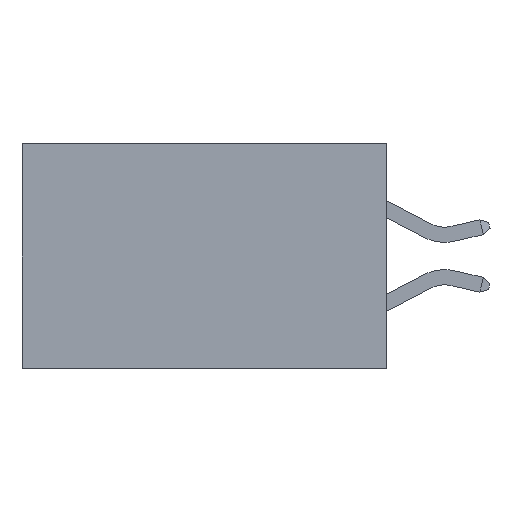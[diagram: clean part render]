
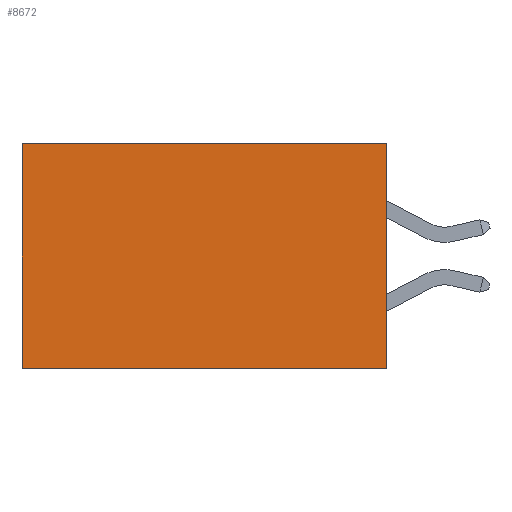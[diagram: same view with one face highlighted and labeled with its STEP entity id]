
A CAD part, left-side view. The second image highlights one B-rep face of the part: STEP entity #8672.
In plain terms, the highlighted planar face has unit normal (-1, 0, 0).
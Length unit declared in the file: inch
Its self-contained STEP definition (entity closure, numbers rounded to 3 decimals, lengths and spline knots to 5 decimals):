
#946 = EDGE_CURVE ( 'NONE', #15210, #5547, #4296, .T. ) ;
#956 = CARTESIAN_POINT ( 'NONE',  ( 0.2615, 0., -0.37 ) ) ;
#988 = DIRECTION ( 'NONE',  ( 0., 1., 0. ) ) ;
#1098 = VECTOR ( 'NONE', #13714, 39.37008 ) ;
#1459 = VERTEX_POINT ( 'NONE', #13126 ) ;
#1573 = CARTESIAN_POINT ( 'NONE',  ( 0.2615, 0., 0. ) ) ;
#2180 = LINE ( 'NONE', #15734, #11172 ) ;
#2649 = EDGE_CURVE ( 'NONE', #1459, #5547, #2180, .T. ) ;
#2965 = LINE ( 'NONE', #1573, #1098 ) ;
#4191 = CARTESIAN_POINT ( 'NONE',  ( 0.2615, 0., -0.37 ) ) ;
#4296 = LINE ( 'NONE', #4191, #9653 ) ;
#5547 = VERTEX_POINT ( 'NONE', #11814 ) ;
#5952 = PLANE ( 'NONE',  #8440 ) ;
#6845 = CARTESIAN_POINT ( 'NONE',  ( 0.2615, 0., -0.37 ) ) ;
#7535 = EDGE_CURVE ( 'NONE', #8858, #15210, #12369, .T. ) ;
#8304 = ORIENTED_EDGE ( 'NONE', *, *, #7535, .F. ) ;
#8440 = AXIS2_PLACEMENT_3D ( 'NONE', #956, #8785, #15122 ) ;
#8672 = ADVANCED_FACE ( 'NONE', ( #14727 ), #5952, .F. ) ;
#8690 = VECTOR ( 'NONE', #12749, 39.37008 ) ;
#8785 = DIRECTION ( 'NONE',  ( 1., 0., 0. ) ) ;
#8858 = VERTEX_POINT ( 'NONE', #10401 ) ;
#9235 = ORIENTED_EDGE ( 'NONE', *, *, #946, .F. ) ;
#9653 = VECTOR ( 'NONE', #988, 39.37008 ) ;
#10401 = CARTESIAN_POINT ( 'NONE',  ( 0.2615, 0., 0. ) ) ;
#11172 = VECTOR ( 'NONE', #11224, 39.37008 ) ;
#11224 = DIRECTION ( 'NONE',  ( 0., 0., -1. ) ) ;
#11814 = CARTESIAN_POINT ( 'NONE',  ( 0.2615, 0.6, -0.37 ) ) ;
#11882 = EDGE_LOOP ( 'NONE', ( #16677, #9235, #8304, #14947 ) ) ;
#12369 = LINE ( 'NONE', #12557, #8690 ) ;
#12557 = CARTESIAN_POINT ( 'NONE',  ( 0.2615, 0., -0.37 ) ) ;
#12749 = DIRECTION ( 'NONE',  ( 0., 0., -1. ) ) ;
#13126 = CARTESIAN_POINT ( 'NONE',  ( 0.2615, 0.6, 0. ) ) ;
#13714 = DIRECTION ( 'NONE',  ( 0., 1., 0. ) ) ;
#14727 = FACE_OUTER_BOUND ( 'NONE', #11882, .T. ) ;
#14947 = ORIENTED_EDGE ( 'NONE', *, *, #14963, .T. ) ;
#14963 = EDGE_CURVE ( 'NONE', #8858, #1459, #2965, .T. ) ;
#15122 = DIRECTION ( 'NONE',  ( 0., 0., -1. ) ) ;
#15210 = VERTEX_POINT ( 'NONE', #6845 ) ;
#15734 = CARTESIAN_POINT ( 'NONE',  ( 0.2615, 0.6, -0.37 ) ) ;
#16677 = ORIENTED_EDGE ( 'NONE', *, *, #2649, .T. ) ;
